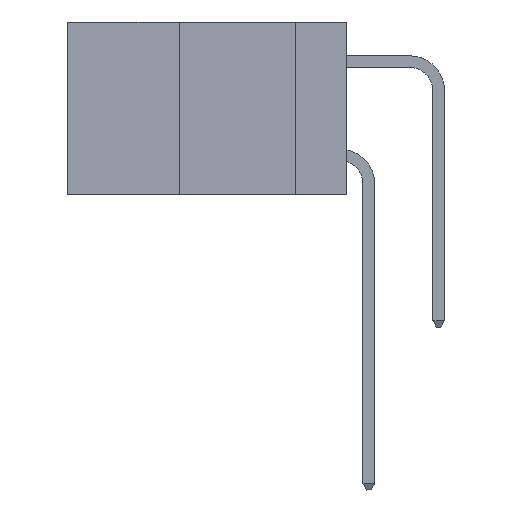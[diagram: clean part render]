
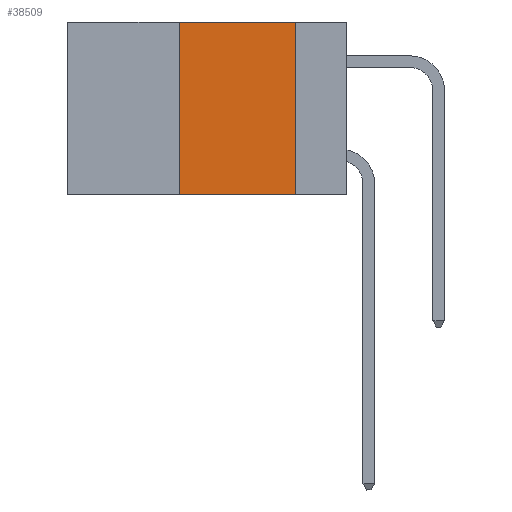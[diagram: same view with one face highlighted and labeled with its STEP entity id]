
A CAD part, left-side view. The second image highlights one B-rep face of the part: STEP entity #38509.
In plain terms, the highlighted planar face has unit normal (-1, 0, 0).
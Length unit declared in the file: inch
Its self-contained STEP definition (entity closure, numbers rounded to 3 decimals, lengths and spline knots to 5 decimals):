
#1137 = VECTOR ( 'NONE', #32880, 39.37008 ) ;
#3203 = DIRECTION ( 'NONE',  ( 0., -1., 0. ) ) ;
#3351 = EDGE_CURVE ( 'NONE', #5514, #35168, #24576, .T. ) ;
#4410 = ORIENTED_EDGE ( 'NONE', *, *, #23485, .F. ) ;
#5056 = CARTESIAN_POINT ( 'NONE',  ( 0., 0.6, 0. ) ) ;
#5155 = VECTOR ( 'NONE', #19295, 39.37008 ) ;
#5514 = VERTEX_POINT ( 'NONE', #22399 ) ;
#5771 = FACE_OUTER_BOUND ( 'NONE', #26812, .T. ) ;
#6252 = LINE ( 'NONE', #10010, #5155 ) ;
#7612 = PLANE ( 'NONE',  #11173 ) ;
#7635 = LINE ( 'NONE', #12758, #44144 ) ;
#7660 = VECTOR ( 'NONE', #3203, 39.37008 ) ;
#10010 = CARTESIAN_POINT ( 'NONE',  ( 0., 0.36, 0. ) ) ;
#11173 = AXIS2_PLACEMENT_3D ( 'NONE', #41915, #21162, #35455 ) ;
#11876 = CARTESIAN_POINT ( 'NONE',  ( 0., 0.36, -0.37 ) ) ;
#12758 = CARTESIAN_POINT ( 'NONE',  ( 0., 0.11, 0. ) ) ;
#17958 = EDGE_CURVE ( 'NONE', #35168, #23478, #7635, .T. ) ;
#19295 = DIRECTION ( 'NONE',  ( 0., 0., 1. ) ) ;
#21162 = DIRECTION ( 'NONE',  ( 1., 0., 0. ) ) ;
#22399 = CARTESIAN_POINT ( 'NONE',  ( 0., 0.36, 0. ) ) ;
#22646 = VERTEX_POINT ( 'NONE', #11876 ) ;
#23478 = VERTEX_POINT ( 'NONE', #33425 ) ;
#23485 = EDGE_CURVE ( 'NONE', #22646, #5514, #6252, .T. ) ;
#24576 = LINE ( 'NONE', #5056, #1137 ) ;
#26159 = LINE ( 'NONE', #44978, #7660 ) ;
#26812 = EDGE_LOOP ( 'NONE', ( #44985, #36182, #4410, #28129 ) ) ;
#28129 = ORIENTED_EDGE ( 'NONE', *, *, #42077, .T. ) ;
#32379 = CARTESIAN_POINT ( 'NONE',  ( 0., 0.11, 0. ) ) ;
#32880 = DIRECTION ( 'NONE',  ( 0., -1., 0. ) ) ;
#33425 = CARTESIAN_POINT ( 'NONE',  ( 0., 0.11, -0.37 ) ) ;
#35168 = VERTEX_POINT ( 'NONE', #32379 ) ;
#35455 = DIRECTION ( 'NONE',  ( 0., 0., -1. ) ) ;
#36182 = ORIENTED_EDGE ( 'NONE', *, *, #3351, .F. ) ;
#38509 = ADVANCED_FACE ( 'NONE', ( #5771 ), #7612, .F. ) ;
#41915 = CARTESIAN_POINT ( 'NONE',  ( 0., 0.6, 0. ) ) ;
#42077 = EDGE_CURVE ( 'NONE', #22646, #23478, #26159, .T. ) ;
#43857 = DIRECTION ( 'NONE',  ( 0., 0., -1. ) ) ;
#44144 = VECTOR ( 'NONE', #43857, 39.37008 ) ;
#44978 = CARTESIAN_POINT ( 'NONE',  ( 0., 0.6, -0.37 ) ) ;
#44985 = ORIENTED_EDGE ( 'NONE', *, *, #17958, .F. ) ;
